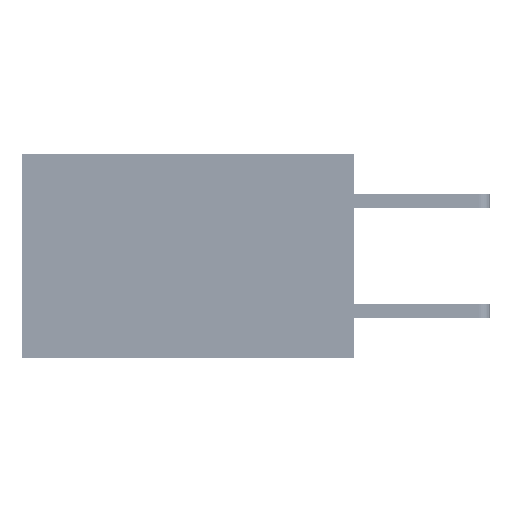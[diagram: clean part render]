
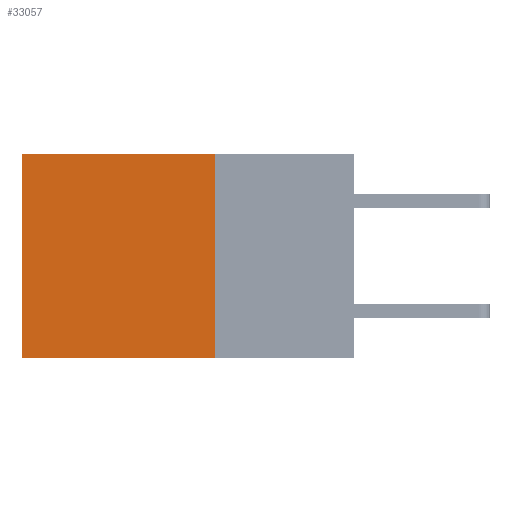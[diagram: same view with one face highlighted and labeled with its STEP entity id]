
A CAD part, left-side view. The second image highlights one B-rep face of the part: STEP entity #33057.
In plain terms, the highlighted planar face has unit normal (-1, 0, 0).
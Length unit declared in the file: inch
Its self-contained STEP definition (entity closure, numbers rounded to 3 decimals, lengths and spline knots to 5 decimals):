
#88 = CARTESIAN_POINT ( 'NONE',  ( 0.2875, 0.6, -0.37 ) ) ;
#305 = VERTEX_POINT ( 'NONE', #42163 ) ;
#2309 = DIRECTION ( 'NONE',  ( 0., 1., 0. ) ) ;
#2450 = VERTEX_POINT ( 'NONE', #48973 ) ;
#3006 = LINE ( 'NONE', #48617, #24618 ) ;
#4680 = DIRECTION ( 'NONE',  ( 0., 0., -1. ) ) ;
#6115 = CARTESIAN_POINT ( 'NONE',  ( 0.2875, 0.25, 0. ) ) ;
#11812 = EDGE_CURVE ( 'NONE', #33513, #2450, #40752, .T. ) ;
#12250 = CARTESIAN_POINT ( 'NONE',  ( 0.2875, 0.6, 0. ) ) ;
#14258 = ORIENTED_EDGE ( 'NONE', *, *, #17371, .T. ) ;
#17371 = EDGE_CURVE ( 'NONE', #2450, #31053, #42726, .T. ) ;
#18147 = DIRECTION ( 'NONE',  ( 1., 0., 0. ) ) ;
#19344 = CARTESIAN_POINT ( 'NONE',  ( 0.2875, 0.25, -0.37 ) ) ;
#19827 = ORIENTED_EDGE ( 'NONE', *, *, #38555, .F. ) ;
#24618 = VECTOR ( 'NONE', #32723, 39.37008 ) ;
#25388 = CARTESIAN_POINT ( 'NONE',  ( 0.2875, 0.25, 0. ) ) ;
#26712 = LINE ( 'NONE', #19344, #29798 ) ;
#27100 = ORIENTED_EDGE ( 'NONE', *, *, #47719, .F. ) ;
#29798 = VECTOR ( 'NONE', #31614, 39.37008 ) ;
#31053 = VERTEX_POINT ( 'NONE', #88 ) ;
#31491 = VECTOR ( 'NONE', #2309, 39.37008 ) ;
#31614 = DIRECTION ( 'NONE',  ( 0., 1., 0. ) ) ;
#32723 = DIRECTION ( 'NONE',  ( 0., 0., -1. ) ) ;
#33057 = ADVANCED_FACE ( 'NONE', ( #37063 ), #41805, .F. ) ;
#33513 = VERTEX_POINT ( 'NONE', #25388 ) ;
#37063 = FACE_OUTER_BOUND ( 'NONE', #38036, .T. ) ;
#38036 = EDGE_LOOP ( 'NONE', ( #14258, #19827, #27100, #44671 ) ) ;
#38340 = CARTESIAN_POINT ( 'NONE',  ( 0.2875, 0.25, 0. ) ) ;
#38555 = EDGE_CURVE ( 'NONE', #305, #31053, #26712, .T. ) ;
#39860 = AXIS2_PLACEMENT_3D ( 'NONE', #38340, #18147, #45802 ) ;
#40752 = LINE ( 'NONE', #6115, #31491 ) ;
#41805 = PLANE ( 'NONE',  #39860 ) ;
#42163 = CARTESIAN_POINT ( 'NONE',  ( 0.2875, 0.25, -0.37 ) ) ;
#42726 = LINE ( 'NONE', #12250, #46452 ) ;
#44671 = ORIENTED_EDGE ( 'NONE', *, *, #11812, .T. ) ;
#45802 = DIRECTION ( 'NONE',  ( 0., 0., -1. ) ) ;
#46452 = VECTOR ( 'NONE', #4680, 39.37008 ) ;
#47719 = EDGE_CURVE ( 'NONE', #33513, #305, #3006, .T. ) ;
#48617 = CARTESIAN_POINT ( 'NONE',  ( 0.2875, 0.25, 0. ) ) ;
#48973 = CARTESIAN_POINT ( 'NONE',  ( 0.2875, 0.6, 0. ) ) ;
